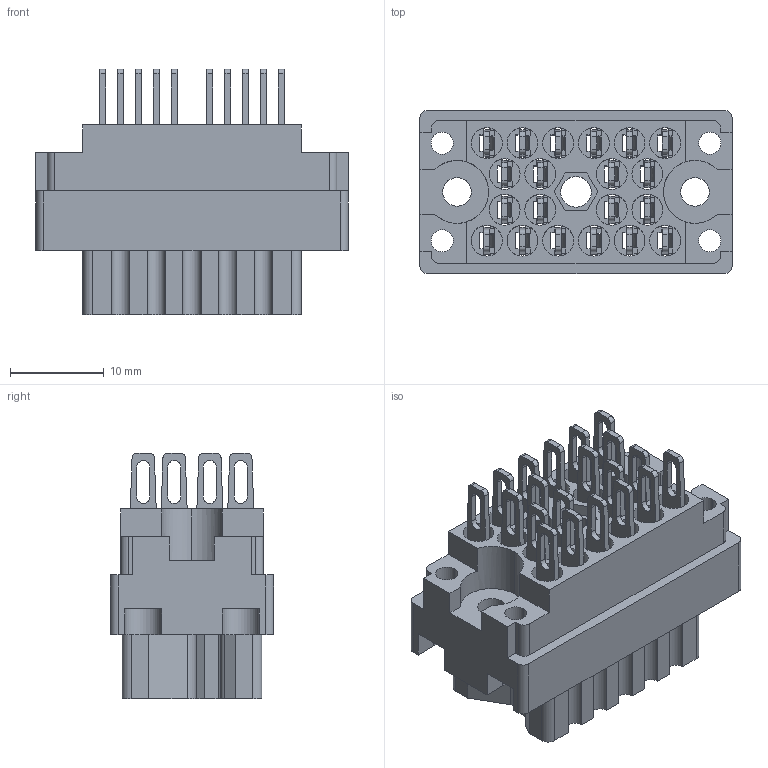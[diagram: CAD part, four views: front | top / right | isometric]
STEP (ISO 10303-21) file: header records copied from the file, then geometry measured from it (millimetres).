
FILE_DESCRIPTION (( 'STEP AP203' ), '1' );
FILE_NAME ('516-020-500-200.STEP', '2020-03-04T17:10:30', ( '' ), ( '' ), 'SwSTEP 2.0', 'SolidWorks 2016', '' );
FILE_SCHEMA (( 'CONFIG_CONTROL_DESIGN' ));
Length unit declared in the file: inch
Products named in the file (3): 516 Part Receptacle_020; 516-292-001_500 Contact; 516-020-500-200
Assembly tree (21 placements, depth 2):
  516-020-500-200
    516 Part Receptacle_020
    516-292-001_500 Contact  x20
Bounding box: 33.32 x 17.42 x 26.21 mm (x, y, z)
Volume: 5750.3 mm3; surface area: 11898.4 mm2
Topology: 21 solids, 21 shells, 2130 faces, 6190 edges, 4112 vertices
Faces by surface type: plane 1275, cylinder 733, bspline 120, cone 2
Entity records: 24008 total; most frequent: CARTESIAN_POINT 4343, ORIENTED_EDGE 4020, DIRECTION 3900, EDGE_CURVE 2010, VECTOR 1460, LINE 1460, VERTEX_POINT 1338, AXIS2_PLACEMENT_3D 1220
